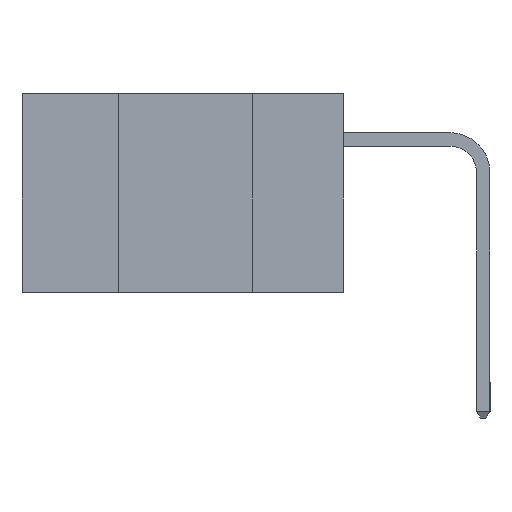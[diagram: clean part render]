
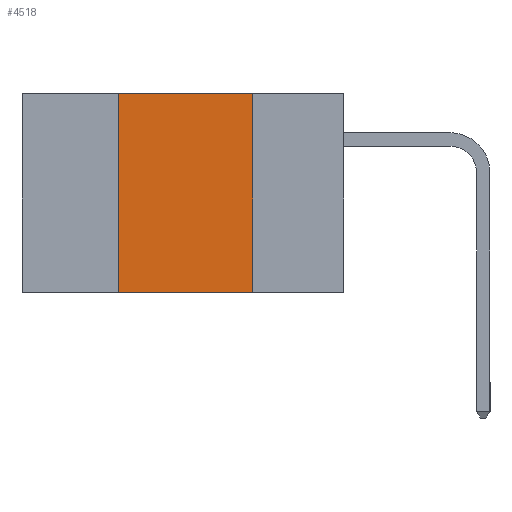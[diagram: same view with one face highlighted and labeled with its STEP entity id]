
A CAD part, left-side view. The second image highlights one B-rep face of the part: STEP entity #4518.
In plain terms, the highlighted planar face has unit normal (-1, 0, 0).
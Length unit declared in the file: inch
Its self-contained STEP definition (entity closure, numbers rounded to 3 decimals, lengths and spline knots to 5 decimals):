
#1952 = DIRECTION ( 'NONE',  ( 0., -1., 0. ) ) ;
#3700 = LINE ( 'NONE', #20861, #15577 ) ;
#4436 = VECTOR ( 'NONE', #20975, 39.37008 ) ;
#4518 = ADVANCED_FACE ( 'NONE', ( #9588 ), #11896, .F. ) ;
#4638 = EDGE_CURVE ( 'NONE', #6762, #8975, #3700, .T. ) ;
#4952 = LINE ( 'NONE', #8502, #4436 ) ;
#5441 = CARTESIAN_POINT ( 'NONE',  ( 0., 0.17, 0. ) ) ;
#5556 = DIRECTION ( 'NONE',  ( 0., -1., 0. ) ) ;
#5673 = EDGE_LOOP ( 'NONE', ( #20135, #18028, #18775, #14525 ) ) ;
#5755 = EDGE_CURVE ( 'NONE', #6762, #6889, #4952, .T. ) ;
#5856 = VECTOR ( 'NONE', #5556, 39.37008 ) ;
#6762 = VERTEX_POINT ( 'NONE', #12922 ) ;
#6889 = VERTEX_POINT ( 'NONE', #9270 ) ;
#7305 = CARTESIAN_POINT ( 'NONE',  ( 0., 0.17, 0. ) ) ;
#7751 = CARTESIAN_POINT ( 'NONE',  ( 0., 0.17, -0.37 ) ) ;
#8038 = DIRECTION ( 'NONE',  ( 1., 0., 0. ) ) ;
#8502 = CARTESIAN_POINT ( 'NONE',  ( 0., 0.42, 0. ) ) ;
#8975 = VERTEX_POINT ( 'NONE', #7751 ) ;
#9270 = CARTESIAN_POINT ( 'NONE',  ( 0., 0.42, 0. ) ) ;
#9588 = FACE_OUTER_BOUND ( 'NONE', #5673, .T. ) ;
#10008 = VERTEX_POINT ( 'NONE', #5441 ) ;
#10104 = EDGE_CURVE ( 'NONE', #10008, #8975, #20157, .T. ) ;
#10608 = VECTOR ( 'NONE', #20137, 39.37008 ) ;
#10945 = DIRECTION ( 'NONE',  ( 0., 0., -1. ) ) ;
#11167 = LINE ( 'NONE', #13598, #5856 ) ;
#11525 = CARTESIAN_POINT ( 'NONE',  ( 0., 0.6, 0. ) ) ;
#11896 = PLANE ( 'NONE',  #19944 ) ;
#12922 = CARTESIAN_POINT ( 'NONE',  ( 0., 0.42, -0.37 ) ) ;
#13598 = CARTESIAN_POINT ( 'NONE',  ( 0., 0.6, 0. ) ) ;
#14525 = ORIENTED_EDGE ( 'NONE', *, *, #4638, .T. ) ;
#15577 = VECTOR ( 'NONE', #1952, 39.37008 ) ;
#18028 = ORIENTED_EDGE ( 'NONE', *, *, #19665, .F. ) ;
#18775 = ORIENTED_EDGE ( 'NONE', *, *, #5755, .F. ) ;
#19665 = EDGE_CURVE ( 'NONE', #6889, #10008, #11167, .T. ) ;
#19944 = AXIS2_PLACEMENT_3D ( 'NONE', #11525, #8038, #10945 ) ;
#20135 = ORIENTED_EDGE ( 'NONE', *, *, #10104, .F. ) ;
#20137 = DIRECTION ( 'NONE',  ( 0., 0., -1. ) ) ;
#20157 = LINE ( 'NONE', #7305, #10608 ) ;
#20861 = CARTESIAN_POINT ( 'NONE',  ( 0., 0.6, -0.37 ) ) ;
#20975 = DIRECTION ( 'NONE',  ( 0., 0., 1. ) ) ;
